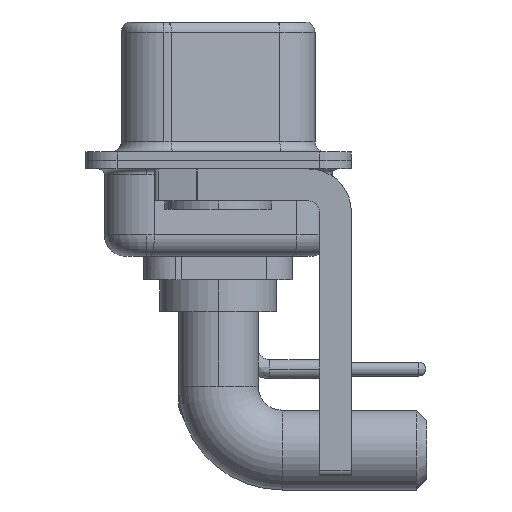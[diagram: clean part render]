
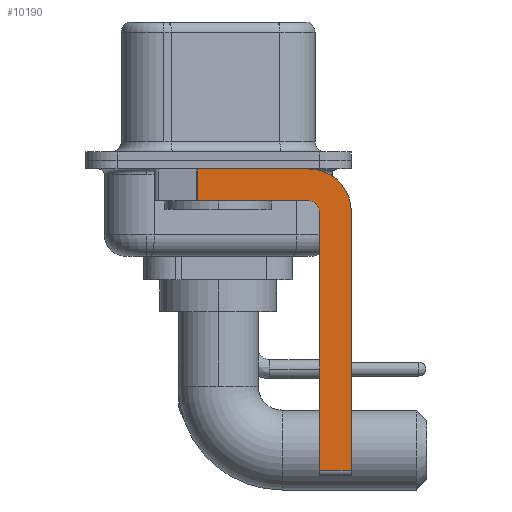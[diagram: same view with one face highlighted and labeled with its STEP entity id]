
A CAD part, left-side view. The second image highlights one B-rep face of the part: STEP entity #10190.
In plain terms, the highlighted planar face has unit normal (-1, 0, 0).
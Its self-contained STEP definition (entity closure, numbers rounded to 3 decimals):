
#269 = DIRECTION ( 'NONE',  ( 0., 0., -1. ) ) ;
#310 = DIRECTION ( 'NONE',  ( 0., 0., -1. ) ) ;
#517 = EDGE_CURVE ( 'NONE', #17349, #17369, #10093, .T. ) ;
#1002 = DIRECTION ( 'NONE',  ( 0., 0., -1. ) ) ;
#1664 = EDGE_CURVE ( 'NONE', #17005, #21619, #6411, .T. ) ;
#2782 = DIRECTION ( 'NONE',  ( 0., 0., 1. ) ) ;
#2790 = AXIS2_PLACEMENT_3D ( 'NONE', #22016, #2960, #20030 ) ;
#2960 = DIRECTION ( 'NONE',  ( 1., 0., 0. ) ) ;
#3095 = DIRECTION ( 'NONE',  ( 1., 0., 0. ) ) ;
#3764 = VECTOR ( 'NONE', #15162, 1000. ) ;
#4131 = CIRCLE ( 'NONE', #25927, 2. ) ;
#4354 = LINE ( 'NONE', #11009, #10043 ) ;
#4930 = CARTESIAN_POINT ( 'NONE',  ( -2.9, -4.75, -14.55 ) ) ;
#4943 = ORIENTED_EDGE ( 'NONE', *, *, #22653, .F. ) ;
#5024 = CARTESIAN_POINT ( 'NONE',  ( -2.9, -4.25, -0.4 ) ) ;
#5465 = VECTOR ( 'NONE', #7417, 1000. ) ;
#5599 = FACE_OUTER_BOUND ( 'NONE', #10390, .T. ) ;
#5908 = ORIENTED_EDGE ( 'NONE', *, *, #12705, .T. ) ;
#6411 = LINE ( 'NONE', #8342, #3764 ) ;
#7291 = VECTOR ( 'NONE', #16219, 1000. ) ;
#7417 = DIRECTION ( 'NONE',  ( 0., -1., 0. ) ) ;
#8290 = ORIENTED_EDGE ( 'NONE', *, *, #19581, .F. ) ;
#8342 = CARTESIAN_POINT ( 'NONE',  ( -2.9, -4.25, -1.9 ) ) ;
#8642 = EDGE_CURVE ( 'NONE', #14068, #16187, #17825, .T. ) ;
#8675 = EDGE_CURVE ( 'NONE', #16187, #20718, #4131, .T. ) ;
#9807 = CARTESIAN_POINT ( 'NONE',  ( -2.9, -4.25, -1.9 ) ) ;
#9922 = DIRECTION ( 'NONE',  ( -1., 0., 0. ) ) ;
#10043 = VECTOR ( 'NONE', #310, 1000. ) ;
#10093 = LINE ( 'NONE', #20389, #7291 ) ;
#10190 = ADVANCED_FACE ( 'NONE', ( #5599 ), #11290, .F. ) ;
#10390 = EDGE_LOOP ( 'NONE', ( #16081, #5908, #14661, #20423, #8290, #22455, #4943, #18466 ) ) ;
#11009 = CARTESIAN_POINT ( 'NONE',  ( -2.9, -6.25, -2.4 ) ) ;
#11290 = PLANE ( 'NONE',  #2790 ) ;
#12705 = EDGE_CURVE ( 'NONE', #14068, #21619, #25961, .T. ) ;
#13428 = CIRCLE ( 'NONE', #20517, 0.5 ) ;
#13779 = VERTEX_POINT ( 'NONE', #17677 ) ;
#14068 = VERTEX_POINT ( 'NONE', #23079 ) ;
#14661 = ORIENTED_EDGE ( 'NONE', *, *, #1664, .F. ) ;
#15162 = DIRECTION ( 'NONE',  ( 0., 1., 0. ) ) ;
#16007 = CARTESIAN_POINT ( 'NONE',  ( -2.9, -6.25, -2.4 ) ) ;
#16009 = CARTESIAN_POINT ( 'NONE',  ( -2.9, -4.25, -2.4 ) ) ;
#16081 = ORIENTED_EDGE ( 'NONE', *, *, #8642, .F. ) ;
#16187 = VERTEX_POINT ( 'NONE', #5024 ) ;
#16219 = DIRECTION ( 'NONE',  ( 0., -1., 0. ) ) ;
#16368 = VECTOR ( 'NONE', #269, 1000. ) ;
#17005 = VERTEX_POINT ( 'NONE', #9807 ) ;
#17349 = VERTEX_POINT ( 'NONE', #4930 ) ;
#17369 = VERTEX_POINT ( 'NONE', #24144 ) ;
#17433 = EDGE_CURVE ( 'NONE', #13779, #17005, #13428, .T. ) ;
#17677 = CARTESIAN_POINT ( 'NONE',  ( -2.9, -4.75, -2.4 ) ) ;
#17825 = LINE ( 'NONE', #26352, #5465 ) ;
#18411 = VECTOR ( 'NONE', #2782, 1000. ) ;
#18466 = ORIENTED_EDGE ( 'NONE', *, *, #8675, .F. ) ;
#19317 = CARTESIAN_POINT ( 'NONE',  ( -2.9, 0.978, -1.9 ) ) ;
#19581 = EDGE_CURVE ( 'NONE', #17349, #13779, #21681, .T. ) ;
#20030 = DIRECTION ( 'NONE',  ( 0., 0., -1. ) ) ;
#20389 = CARTESIAN_POINT ( 'NONE',  ( -2.9, -4.25, -14.55 ) ) ;
#20423 = ORIENTED_EDGE ( 'NONE', *, *, #17433, .F. ) ;
#20517 = AXIS2_PLACEMENT_3D ( 'NONE', #24823, #9922, #22317 ) ;
#20718 = VERTEX_POINT ( 'NONE', #16007 ) ;
#21619 = VERTEX_POINT ( 'NONE', #24911 ) ;
#21681 = LINE ( 'NONE', #26173, #18411 ) ;
#22016 = CARTESIAN_POINT ( 'NONE',  ( -2.9, -4.25, -2.4 ) ) ;
#22317 = DIRECTION ( 'NONE',  ( 0., 0., 1. ) ) ;
#22455 = ORIENTED_EDGE ( 'NONE', *, *, #517, .T. ) ;
#22653 = EDGE_CURVE ( 'NONE', #20718, #17369, #4354, .T. ) ;
#23079 = CARTESIAN_POINT ( 'NONE',  ( -2.9, 0.978, -0.4 ) ) ;
#24144 = CARTESIAN_POINT ( 'NONE',  ( -2.9, -6.25, -14.55 ) ) ;
#24823 = CARTESIAN_POINT ( 'NONE',  ( -2.9, -4.25, -2.4 ) ) ;
#24911 = CARTESIAN_POINT ( 'NONE',  ( -2.9, 0.978, -1.9 ) ) ;
#25927 = AXIS2_PLACEMENT_3D ( 'NONE', #16009, #3095, #1002 ) ;
#25961 = LINE ( 'NONE', #19317, #16368 ) ;
#26173 = CARTESIAN_POINT ( 'NONE',  ( -2.9, -4.75, -14.8 ) ) ;
#26352 = CARTESIAN_POINT ( 'NONE',  ( -2.9, 3., -0.4 ) ) ;
